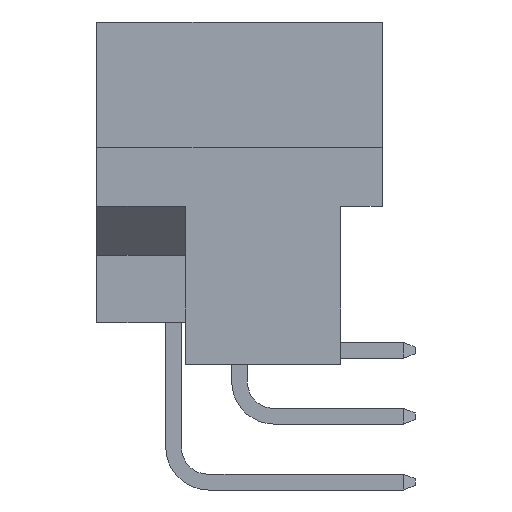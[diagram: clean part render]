
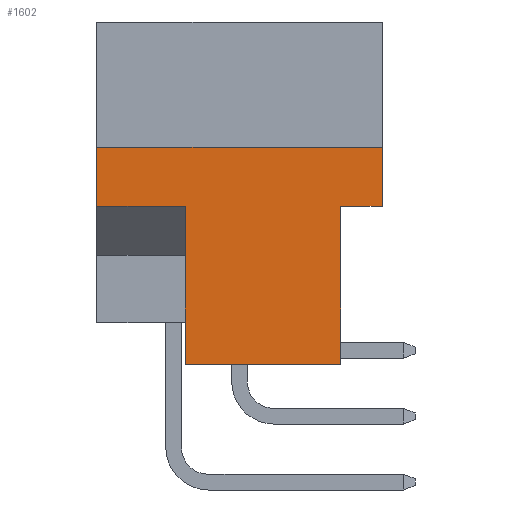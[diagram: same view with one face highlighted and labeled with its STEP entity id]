
A CAD part, left-side view. The second image highlights one B-rep face of the part: STEP entity #1602.
In plain terms, the highlighted planar face has unit normal (-1, 0, 0).
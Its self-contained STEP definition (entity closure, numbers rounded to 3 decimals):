
#10 = EDGE_CURVE ( 'NONE', #1410, #5675, #2212, .T. ) ;
#108 = CARTESIAN_POINT ( 'NONE',  ( 0., 0., 0. ) ) ;
#207 = CARTESIAN_POINT ( 'NONE',  ( 0., 10.998, -4.826 ) ) ;
#212 = VERTEX_POINT ( 'NONE', #6064 ) ;
#279 = ORIENTED_EDGE ( 'NONE', *, *, #6202, .F. ) ;
#592 = CARTESIAN_POINT ( 'NONE',  ( 0., 7.597, -7.112 ) ) ;
#867 = ORIENTED_EDGE ( 'NONE', *, *, #4986, .F. ) ;
#923 = ORIENTED_EDGE ( 'NONE', *, *, #2608, .F. ) ;
#960 = CARTESIAN_POINT ( 'NONE',  ( 0., 7.597, -13.2 ) ) ;
#1350 = LINE ( 'NONE', #108, #3989 ) ;
#1403 = VECTOR ( 'NONE', #2155, 1000. ) ;
#1410 = VERTEX_POINT ( 'NONE', #3348 ) ;
#1419 = CARTESIAN_POINT ( 'NONE',  ( 0., 0., -7.112 ) ) ;
#1463 = DIRECTION ( 'NONE',  ( 0., 0., -1. ) ) ;
#1530 = VERTEX_POINT ( 'NONE', #6359 ) ;
#1602 = ADVANCED_FACE ( 'NONE', ( #4670 ), #5696, .F. ) ;
#1605 = ORIENTED_EDGE ( 'NONE', *, *, #6896, .T. ) ;
#1933 = VECTOR ( 'NONE', #5084, 1000. ) ;
#2155 = DIRECTION ( 'NONE',  ( 0., 0., 1. ) ) ;
#2157 = ORIENTED_EDGE ( 'NONE', *, *, #10, .F. ) ;
#2212 = LINE ( 'NONE', #960, #4047 ) ;
#2336 = CARTESIAN_POINT ( 'NONE',  ( 0., 7.597, -7.112 ) ) ;
#2350 = DIRECTION ( 'NONE',  ( 1., 0., 0. ) ) ;
#2374 = LINE ( 'NONE', #592, #4396 ) ;
#2495 = CARTESIAN_POINT ( 'NONE',  ( 0., 10.998, -4.826 ) ) ;
#2608 = EDGE_CURVE ( 'NONE', #4860, #3771, #6035, .T. ) ;
#2681 = CARTESIAN_POINT ( 'NONE',  ( 0., 10.998, 0. ) ) ;
#3348 = CARTESIAN_POINT ( 'NONE',  ( 0., 7.597, -13.2 ) ) ;
#3473 = LINE ( 'NONE', #7456, #1933 ) ;
#3591 = DIRECTION ( 'NONE',  ( 0., 0., 1. ) ) ;
#3771 = VERTEX_POINT ( 'NONE', #5953 ) ;
#3878 = ORIENTED_EDGE ( 'NONE', *, *, #6954, .T. ) ;
#3914 = CARTESIAN_POINT ( 'NONE',  ( 0., 0., -7.112 ) ) ;
#3989 = VECTOR ( 'NONE', #3591, 1000. ) ;
#4047 = VECTOR ( 'NONE', #6292, 1000. ) ;
#4108 = VERTEX_POINT ( 'NONE', #2495 ) ;
#4269 = EDGE_CURVE ( 'NONE', #212, #4108, #6126, .T. ) ;
#4293 = LINE ( 'NONE', #1419, #4585 ) ;
#4297 = VECTOR ( 'NONE', #1463, 1000. ) ;
#4344 = ORIENTED_EDGE ( 'NONE', *, *, #7365, .F. ) ;
#4396 = VECTOR ( 'NONE', #4688, 1000. ) ;
#4585 = VECTOR ( 'NONE', #6031, 1000. ) ;
#4670 = FACE_OUTER_BOUND ( 'NONE', #6155, .T. ) ;
#4688 = DIRECTION ( 'NONE',  ( 0., 1., 0. ) ) ;
#4860 = VERTEX_POINT ( 'NONE', #6297 ) ;
#4986 = EDGE_CURVE ( 'NONE', #4108, #1530, #7167, .T. ) ;
#5084 = DIRECTION ( 'NONE',  ( 0., -1., 0. ) ) ;
#5437 = DIRECTION ( 'NONE',  ( 0., -1., 0. ) ) ;
#5675 = VERTEX_POINT ( 'NONE', #2336 ) ;
#5696 = PLANE ( 'NONE',  #6050 ) ;
#5767 = CARTESIAN_POINT ( 'NONE',  ( 0., 10.998, 0. ) ) ;
#5943 = ORIENTED_EDGE ( 'NONE', *, *, #4269, .F. ) ;
#5953 = CARTESIAN_POINT ( 'NONE',  ( 0., 1.6, -13.2 ) ) ;
#6031 = DIRECTION ( 'NONE',  ( 0., 1., 0. ) ) ;
#6035 = LINE ( 'NONE', #6643, #4297 ) ;
#6050 = AXIS2_PLACEMENT_3D ( 'NONE', #5767, #2350, #6971 ) ;
#6064 = CARTESIAN_POINT ( 'NONE',  ( 0., 10.998, -7.112 ) ) ;
#6126 = LINE ( 'NONE', #2681, #1403 ) ;
#6155 = EDGE_LOOP ( 'NONE', ( #923, #279, #3878, #867, #5943, #4344, #2157, #1605 ) ) ;
#6202 = EDGE_CURVE ( 'NONE', #6274, #4860, #4293, .T. ) ;
#6274 = VERTEX_POINT ( 'NONE', #3914 ) ;
#6292 = DIRECTION ( 'NONE',  ( 0., 0., 1. ) ) ;
#6297 = CARTESIAN_POINT ( 'NONE',  ( 0., 1.6, -7.112 ) ) ;
#6359 = CARTESIAN_POINT ( 'NONE',  ( 0., 0., -4.826 ) ) ;
#6456 = VECTOR ( 'NONE', #5437, 1000. ) ;
#6643 = CARTESIAN_POINT ( 'NONE',  ( 0., 1.6, 31.022 ) ) ;
#6896 = EDGE_CURVE ( 'NONE', #1410, #3771, #3473, .T. ) ;
#6954 = EDGE_CURVE ( 'NONE', #6274, #1530, #1350, .T. ) ;
#6971 = DIRECTION ( 'NONE',  ( 0., 0., -1. ) ) ;
#7167 = LINE ( 'NONE', #207, #6456 ) ;
#7365 = EDGE_CURVE ( 'NONE', #5675, #212, #2374, .T. ) ;
#7456 = CARTESIAN_POINT ( 'NONE',  ( 0., 10.998, -13.2 ) ) ;
